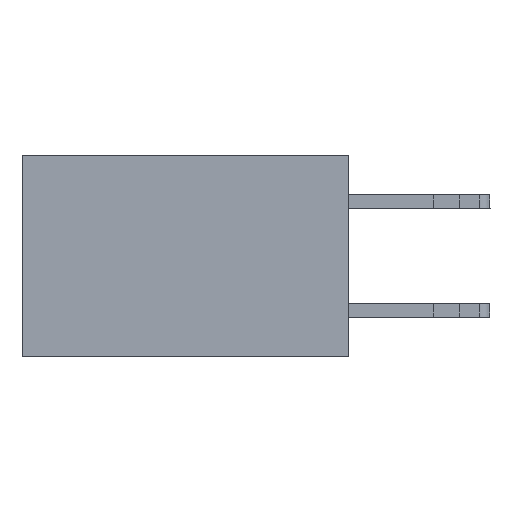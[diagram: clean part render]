
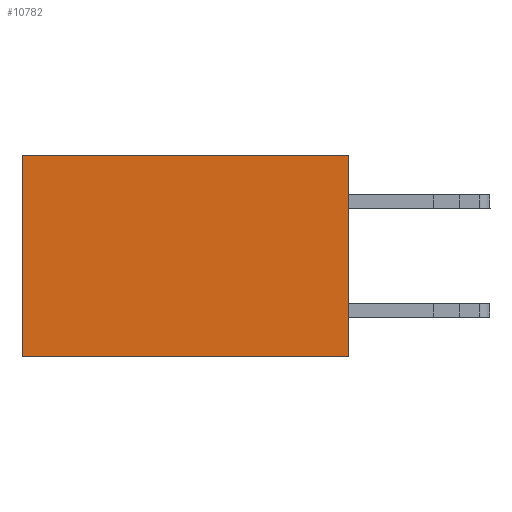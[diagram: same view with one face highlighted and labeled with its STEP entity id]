
A CAD part, left-side view. The second image highlights one B-rep face of the part: STEP entity #10782.
In plain terms, the highlighted planar face has unit normal (-1, 0, 0).
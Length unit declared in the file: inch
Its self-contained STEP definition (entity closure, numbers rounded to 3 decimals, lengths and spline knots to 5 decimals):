
#887 = CARTESIAN_POINT ( 'NONE',  ( 0.2615, 0., -0.37 ) ) ;
#1013 = CARTESIAN_POINT ( 'NONE',  ( 0.2615, 0.6, 0. ) ) ;
#1095 = EDGE_LOOP ( 'NONE', ( #16242, #3230, #16364, #23176 ) ) ;
#1366 = LINE ( 'NONE', #2913, #20967 ) ;
#1382 = VECTOR ( 'NONE', #13679, 39.37008 ) ;
#2044 = DIRECTION ( 'NONE',  ( 0., 0., -1. ) ) ;
#2913 = CARTESIAN_POINT ( 'NONE',  ( 0.2615, 0.6, -0.37 ) ) ;
#3230 = ORIENTED_EDGE ( 'NONE', *, *, #5139, .F. ) ;
#3392 = FACE_OUTER_BOUND ( 'NONE', #1095, .T. ) ;
#4224 = CARTESIAN_POINT ( 'NONE',  ( 0.2615, 0., 0. ) ) ;
#4947 = DIRECTION ( 'NONE',  ( 1., 0., 0. ) ) ;
#5139 = EDGE_CURVE ( 'NONE', #19328, #13010, #22640, .T. ) ;
#6379 = CARTESIAN_POINT ( 'NONE',  ( 0.2615, 0., -0.37 ) ) ;
#6823 = EDGE_CURVE ( 'NONE', #15740, #19328, #18447, .T. ) ;
#6982 = PLANE ( 'NONE',  #7620 ) ;
#7620 = AXIS2_PLACEMENT_3D ( 'NONE', #8890, #4947, #21586 ) ;
#8542 = CARTESIAN_POINT ( 'NONE',  ( 0.2615, 0.6, -0.37 ) ) ;
#8890 = CARTESIAN_POINT ( 'NONE',  ( 0.2615, 0., -0.37 ) ) ;
#9453 = EDGE_CURVE ( 'NONE', #10760, #13010, #1366, .T. ) ;
#10250 = CARTESIAN_POINT ( 'NONE',  ( 0.2615, 0., 0. ) ) ;
#10760 = VERTEX_POINT ( 'NONE', #1013 ) ;
#10782 = ADVANCED_FACE ( 'NONE', ( #3392 ), #6982, .F. ) ;
#12321 = VECTOR ( 'NONE', #2044, 39.37008 ) ;
#13010 = VERTEX_POINT ( 'NONE', #8542 ) ;
#13679 = DIRECTION ( 'NONE',  ( 0., 1., 0. ) ) ;
#14513 = CARTESIAN_POINT ( 'NONE',  ( 0.2615, 0., -0.37 ) ) ;
#14777 = DIRECTION ( 'NONE',  ( 0., 1., 0. ) ) ;
#15000 = LINE ( 'NONE', #4224, #20058 ) ;
#15740 = VERTEX_POINT ( 'NONE', #10250 ) ;
#16242 = ORIENTED_EDGE ( 'NONE', *, *, #9453, .T. ) ;
#16364 = ORIENTED_EDGE ( 'NONE', *, *, #6823, .F. ) ;
#17993 = DIRECTION ( 'NONE',  ( 0., 0., -1. ) ) ;
#18447 = LINE ( 'NONE', #14513, #12321 ) ;
#19328 = VERTEX_POINT ( 'NONE', #887 ) ;
#19646 = EDGE_CURVE ( 'NONE', #15740, #10760, #15000, .T. ) ;
#20058 = VECTOR ( 'NONE', #14777, 39.37008 ) ;
#20967 = VECTOR ( 'NONE', #17993, 39.37008 ) ;
#21586 = DIRECTION ( 'NONE',  ( 0., 0., -1. ) ) ;
#22640 = LINE ( 'NONE', #6379, #1382 ) ;
#23176 = ORIENTED_EDGE ( 'NONE', *, *, #19646, .T. ) ;
